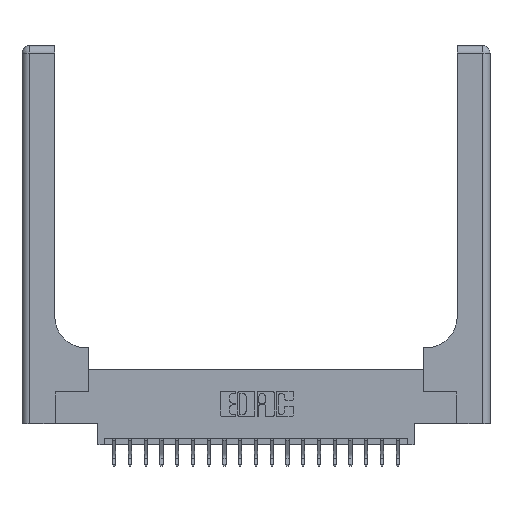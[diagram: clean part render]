
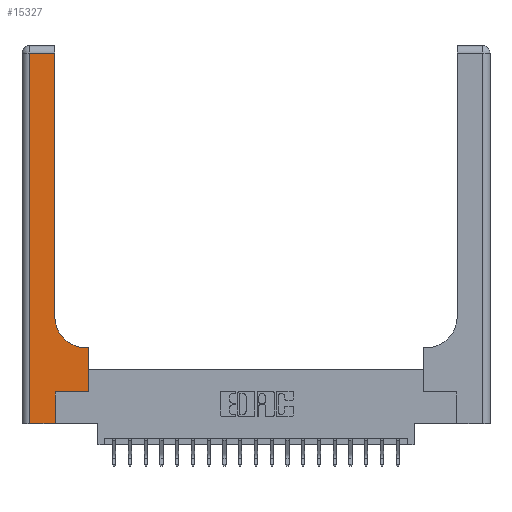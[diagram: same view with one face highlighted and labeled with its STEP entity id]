
A CAD part, top view. The second image highlights one B-rep face of the part: STEP entity #15327.
In plain terms, the highlighted planar face has unit normal (0, 0, 1).
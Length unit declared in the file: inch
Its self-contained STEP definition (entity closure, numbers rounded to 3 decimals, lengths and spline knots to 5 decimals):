
#160 = CARTESIAN_POINT ( 'NONE',  ( 0.528, 0.6, 0.37 ) ) ;
#295 = AXIS2_PLACEMENT_3D ( 'NONE', #10017, #1737, #13238 ) ;
#1103 = ORIENTED_EDGE ( 'NONE', *, *, #12416, .T. ) ;
#1353 = EDGE_CURVE ( 'NONE', #13518, #4016, #15194, .T. ) ;
#1582 = LINE ( 'NONE', #8933, #10920 ) ;
#1636 = EDGE_CURVE ( 'NONE', #4016, #2131, #10681, .T. ) ;
#1737 = DIRECTION ( 'NONE',  ( 0., 0., -1. ) ) ;
#2131 = VERTEX_POINT ( 'NONE', #160 ) ;
#3315 = CARTESIAN_POINT ( 'NONE',  ( 0.51, 0.6, 0.37 ) ) ;
#3357 = ORIENTED_EDGE ( 'NONE', *, *, #5594, .T. ) ;
#3767 = CARTESIAN_POINT ( 'NONE',  ( 0., 0., 0.37 ) ) ;
#3846 = CARTESIAN_POINT ( 'NONE',  ( 0.528, 0.25, 0.37 ) ) ;
#4016 = VERTEX_POINT ( 'NONE', #9506 ) ;
#4072 = ORIENTED_EDGE ( 'NONE', *, *, #13119, .T. ) ;
#4256 = CARTESIAN_POINT ( 'NONE',  ( 0.06, 3., 0.37 ) ) ;
#4299 = VERTEX_POINT ( 'NONE', #5159 ) ;
#4632 = VERTEX_POINT ( 'NONE', #19081 ) ;
#5053 = LINE ( 'NONE', #16196, #8987 ) ;
#5159 = CARTESIAN_POINT ( 'NONE',  ( 0.26, 2.94, 0.37 ) ) ;
#5286 = VECTOR ( 'NONE', #18196, 39.37008 ) ;
#5491 = VECTOR ( 'NONE', #18922, 39.37008 ) ;
#5594 = EDGE_CURVE ( 'NONE', #7311, #4299, #1582, .T. ) ;
#5971 = VERTEX_POINT ( 'NONE', #11465 ) ;
#6420 = DIRECTION ( 'NONE',  ( 1., 0., 0. ) ) ;
#6471 = DIRECTION ( 'NONE',  ( -1., 0., 0. ) ) ;
#6699 = CARTESIAN_POINT ( 'NONE',  ( 0.51, 0.85, 0.37 ) ) ;
#7311 = VERTEX_POINT ( 'NONE', #7433 ) ;
#7433 = CARTESIAN_POINT ( 'NONE',  ( 0.26, 0.85, 0.37 ) ) ;
#7674 = ORIENTED_EDGE ( 'NONE', *, *, #11237, .T. ) ;
#8005 = VECTOR ( 'NONE', #19236, 39.37008 ) ;
#8140 = ORIENTED_EDGE ( 'NONE', *, *, #15312, .T. ) ;
#8379 = DIRECTION ( 'NONE',  ( 1., 0., 0. ) ) ;
#8523 = ORIENTED_EDGE ( 'NONE', *, *, #1636, .T. ) ;
#8933 = CARTESIAN_POINT ( 'NONE',  ( 0.26, 3., 0.37 ) ) ;
#8987 = VECTOR ( 'NONE', #6471, 39.37008 ) ;
#9506 = CARTESIAN_POINT ( 'NONE',  ( 0.528, 0.25, 0.37 ) ) ;
#10017 = CARTESIAN_POINT ( 'NONE',  ( 0., 3., 0.37 ) ) ;
#10176 = VECTOR ( 'NONE', #18517, 39.37008 ) ;
#10217 = CARTESIAN_POINT ( 'NONE',  ( 0.26, 0.6, 0.37 ) ) ;
#10417 = EDGE_CURVE ( 'NONE', #4632, #13518, #20822, .T. ) ;
#10681 = LINE ( 'NONE', #3846, #10176 ) ;
#10920 = VECTOR ( 'NONE', #20165, 39.37008 ) ;
#11113 = CARTESIAN_POINT ( 'NONE',  ( 0.265, 0.25, 0.37 ) ) ;
#11237 = EDGE_CURVE ( 'NONE', #12998, #4632, #14773, .T. ) ;
#11465 = CARTESIAN_POINT ( 'NONE',  ( 0.06, 2.94, 0.37 ) ) ;
#11998 = DIRECTION ( 'NONE',  ( 1., 0., 0. ) ) ;
#12416 = EDGE_CURVE ( 'NONE', #4299, #5971, #5053, .T. ) ;
#12933 = VECTOR ( 'NONE', #6420, 39.37008 ) ;
#12998 = VERTEX_POINT ( 'NONE', #19525 ) ;
#13119 = EDGE_CURVE ( 'NONE', #2131, #19222, #18246, .T. ) ;
#13238 = DIRECTION ( 'NONE',  ( -1., 0., 0. ) ) ;
#13518 = VERTEX_POINT ( 'NONE', #11113 ) ;
#14131 = ORIENTED_EDGE ( 'NONE', *, *, #1353, .T. ) ;
#14295 = VECTOR ( 'NONE', #11998, 39.37008 ) ;
#14749 = EDGE_CURVE ( 'NONE', #5971, #12998, #18440, .T. ) ;
#14773 = LINE ( 'NONE', #3767, #14295 ) ;
#15194 = LINE ( 'NONE', #16138, #12933 ) ;
#15312 = EDGE_CURVE ( 'NONE', #19222, #7311, #19167, .T. ) ;
#15327 = ADVANCED_FACE ( 'NONE', ( #16904 ), #19618, .F. ) ;
#16138 = CARTESIAN_POINT ( 'NONE',  ( 0.265, 0.25, 0.37 ) ) ;
#16196 = CARTESIAN_POINT ( 'NONE',  ( 0., 2.94, 0.37 ) ) ;
#16904 = FACE_OUTER_BOUND ( 'NONE', #20309, .T. ) ;
#17074 = ORIENTED_EDGE ( 'NONE', *, *, #14749, .T. ) ;
#17120 = AXIS2_PLACEMENT_3D ( 'NONE', #6699, #17996, #8379 ) ;
#17336 = CARTESIAN_POINT ( 'NONE',  ( 0.265, 0., 0.37 ) ) ;
#17518 = ORIENTED_EDGE ( 'NONE', *, *, #10417, .T. ) ;
#17996 = DIRECTION ( 'NONE',  ( 0., 0., -1. ) ) ;
#18196 = DIRECTION ( 'NONE',  ( -1., 0., 0. ) ) ;
#18246 = LINE ( 'NONE', #10217, #5286 ) ;
#18440 = LINE ( 'NONE', #4256, #5491 ) ;
#18517 = DIRECTION ( 'NONE',  ( 0., 1., 0. ) ) ;
#18922 = DIRECTION ( 'NONE',  ( 0., -1., 0. ) ) ;
#19081 = CARTESIAN_POINT ( 'NONE',  ( 0.265, 0., 0.37 ) ) ;
#19167 = CIRCLE ( 'NONE', #17120, 0.25 ) ;
#19222 = VERTEX_POINT ( 'NONE', #3315 ) ;
#19236 = DIRECTION ( 'NONE',  ( 0., 1., 0. ) ) ;
#19525 = CARTESIAN_POINT ( 'NONE',  ( 0.06, 0., 0.37 ) ) ;
#19618 = PLANE ( 'NONE',  #295 ) ;
#20165 = DIRECTION ( 'NONE',  ( 0., 1., 0. ) ) ;
#20309 = EDGE_LOOP ( 'NONE', ( #3357, #1103, #17074, #7674, #17518, #14131, #8523, #4072, #8140 ) ) ;
#20822 = LINE ( 'NONE', #17336, #8005 ) ;
